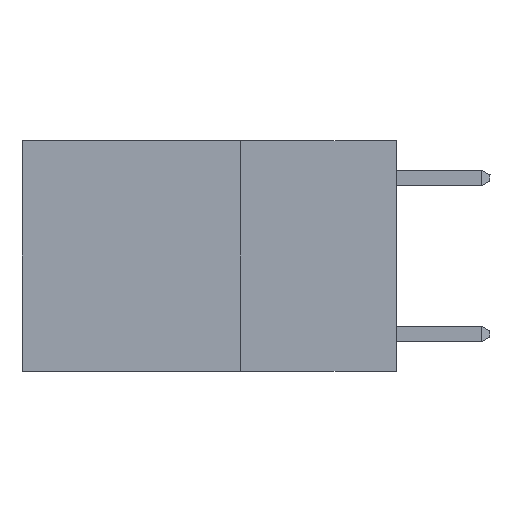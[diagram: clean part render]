
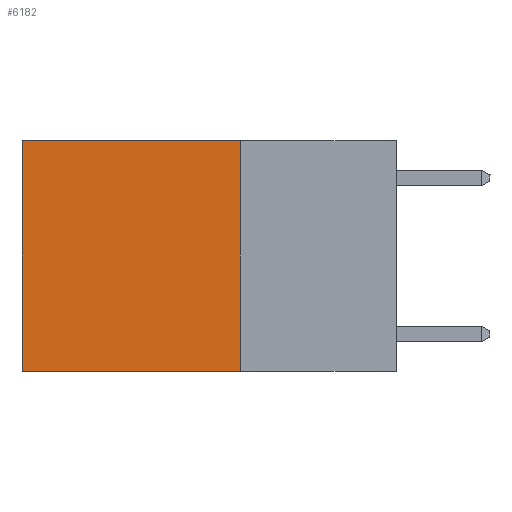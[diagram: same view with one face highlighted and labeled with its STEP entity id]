
A CAD part, left-side view. The second image highlights one B-rep face of the part: STEP entity #6182.
In plain terms, the highlighted planar face has unit normal (-1, 0, 0).
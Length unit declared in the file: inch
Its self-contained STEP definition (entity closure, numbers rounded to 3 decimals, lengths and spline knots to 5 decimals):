
#993 = VECTOR ( 'NONE', #10186, 39.37008 ) ;
#1591 = ORIENTED_EDGE ( 'NONE', *, *, #4378, .F. ) ;
#2163 = LINE ( 'NONE', #2268, #17065 ) ;
#2268 = CARTESIAN_POINT ( 'NONE',  ( 0.2625, 0.25, 0. ) ) ;
#2495 = VECTOR ( 'NONE', #14914, 39.37008 ) ;
#3149 = LINE ( 'NONE', #19108, #993 ) ;
#3514 = DIRECTION ( 'NONE',  ( 0., 0., -1. ) ) ;
#3801 = EDGE_LOOP ( 'NONE', ( #5714, #7883, #1591, #4601 ) ) ;
#4333 = AXIS2_PLACEMENT_3D ( 'NONE', #12253, #19244, #3514 ) ;
#4378 = EDGE_CURVE ( 'NONE', #13012, #7855, #2163, .T. ) ;
#4601 = ORIENTED_EDGE ( 'NONE', *, *, #14287, .T. ) ;
#4650 = CARTESIAN_POINT ( 'NONE',  ( 0.2625, 0.25, -0.37 ) ) ;
#5714 = ORIENTED_EDGE ( 'NONE', *, *, #16138, .T. ) ;
#5835 = VECTOR ( 'NONE', #20381, 39.37008 ) ;
#6182 = ADVANCED_FACE ( 'NONE', ( #7224 ), #14212, .F. ) ;
#6377 = LINE ( 'NONE', #21887, #5835 ) ;
#7224 = FACE_OUTER_BOUND ( 'NONE', #3801, .T. ) ;
#7855 = VERTEX_POINT ( 'NONE', #4650 ) ;
#7883 = ORIENTED_EDGE ( 'NONE', *, *, #21574, .F. ) ;
#8146 = CARTESIAN_POINT ( 'NONE',  ( 0.2625, 0.25, 0. ) ) ;
#10160 = CARTESIAN_POINT ( 'NONE',  ( 0.2625, 0.6, 0. ) ) ;
#10186 = DIRECTION ( 'NONE',  ( 0., 1., 0. ) ) ;
#10791 = DIRECTION ( 'NONE',  ( 0., 0., -1. ) ) ;
#12253 = CARTESIAN_POINT ( 'NONE',  ( 0.2625, 0.25, 0. ) ) ;
#13012 = VERTEX_POINT ( 'NONE', #18020 ) ;
#13209 = LINE ( 'NONE', #8146, #2495 ) ;
#14212 = PLANE ( 'NONE',  #4333 ) ;
#14287 = EDGE_CURVE ( 'NONE', #13012, #21987, #13209, .T. ) ;
#14914 = DIRECTION ( 'NONE',  ( 0., 1., 0. ) ) ;
#16138 = EDGE_CURVE ( 'NONE', #21987, #19992, #6377, .T. ) ;
#16820 = CARTESIAN_POINT ( 'NONE',  ( 0.2625, 0.6, -0.37 ) ) ;
#17065 = VECTOR ( 'NONE', #10791, 39.37008 ) ;
#18020 = CARTESIAN_POINT ( 'NONE',  ( 0.2625, 0.25, 0. ) ) ;
#19108 = CARTESIAN_POINT ( 'NONE',  ( 0.2625, 0.25, -0.37 ) ) ;
#19244 = DIRECTION ( 'NONE',  ( 1., 0., 0. ) ) ;
#19992 = VERTEX_POINT ( 'NONE', #16820 ) ;
#20381 = DIRECTION ( 'NONE',  ( 0., 0., -1. ) ) ;
#21574 = EDGE_CURVE ( 'NONE', #7855, #19992, #3149, .T. ) ;
#21887 = CARTESIAN_POINT ( 'NONE',  ( 0.2625, 0.6, 0. ) ) ;
#21987 = VERTEX_POINT ( 'NONE', #10160 ) ;
